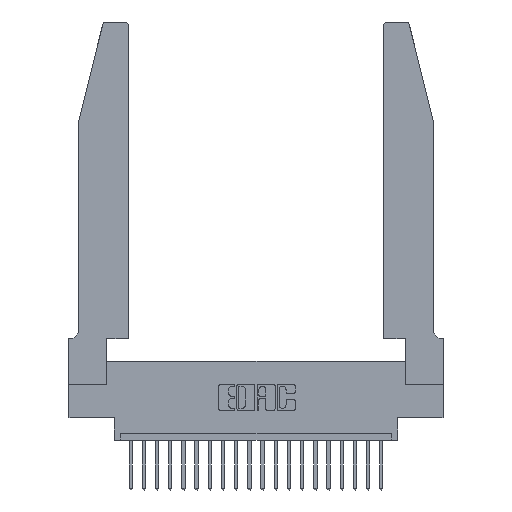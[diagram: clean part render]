
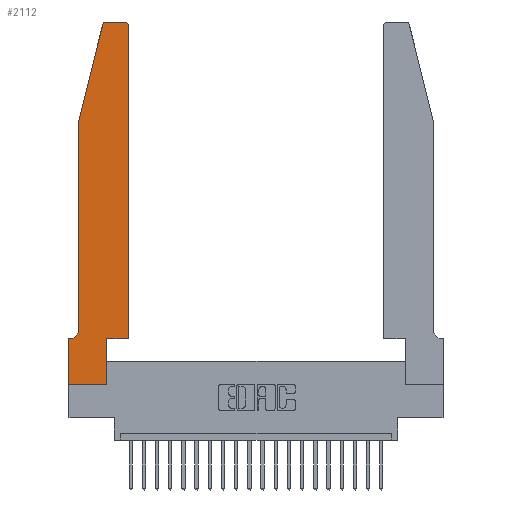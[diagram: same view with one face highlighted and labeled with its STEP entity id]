
A CAD part, top view. The second image highlights one B-rep face of the part: STEP entity #2112.
In plain terms, the highlighted planar face has unit normal (0, 0, 1).
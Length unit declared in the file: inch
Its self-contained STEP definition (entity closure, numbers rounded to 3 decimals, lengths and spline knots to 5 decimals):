
#111 = ORIENTED_EDGE ( 'NONE', *, *, #13829, .T. ) ;
#245 = LINE ( 'NONE', #10132, #5188 ) ;
#274 = CARTESIAN_POINT ( 'NONE',  ( 0.2865, 0., 0.37 ) ) ;
#284 = CIRCLE ( 'NONE', #8115, 0.07 ) ;
#360 = DIRECTION ( 'NONE',  ( -1., 0., 0. ) ) ;
#745 = VERTEX_POINT ( 'NONE', #14329 ) ;
#791 = DIRECTION ( 'NONE',  ( 1., 0., 0. ) ) ;
#1109 = DIRECTION ( 'NONE',  ( 1., 0., 0. ) ) ;
#1461 = CARTESIAN_POINT ( 'NONE',  ( 0.2865, 0.35, 0.37 ) ) ;
#1702 = DIRECTION ( 'NONE',  ( -0.239, -0.971, 0. ) ) ;
#2112 = ADVANCED_FACE ( 'NONE', ( #11909 ), #7901, .T. ) ;
#2151 = DIRECTION ( 'NONE',  ( 0., 1., 0. ) ) ;
#2162 = CARTESIAN_POINT ( 'NONE',  ( 0.25487, 2.72718, 0.37 ) ) ;
#2504 = AXIS2_PLACEMENT_3D ( 'NONE', #12789, #11239, #3029 ) ;
#2702 = VECTOR ( 'NONE', #360, 39.37008 ) ;
#2971 = ORIENTED_EDGE ( 'NONE', *, *, #16387, .T. ) ;
#2990 = CARTESIAN_POINT ( 'NONE',  ( 0.2605, 2.75, 0.37 ) ) ;
#3029 = DIRECTION ( 'NONE',  ( 1., 0., 0. ) ) ;
#3257 = ORIENTED_EDGE ( 'NONE', *, *, #15782, .T. ) ;
#3755 = CARTESIAN_POINT ( 'NONE',  ( 0.4505, 0.35, 0.37 ) ) ;
#3920 = VECTOR ( 'NONE', #17770, 39.37008 ) ;
#4066 = LINE ( 'NONE', #5566, #2702 ) ;
#4079 = LINE ( 'NONE', #17007, #10718 ) ;
#4613 = ORIENTED_EDGE ( 'NONE', *, *, #21035, .T. ) ;
#4940 = CARTESIAN_POINT ( 'NONE',  ( 0., 0.35, 0.37 ) ) ;
#5188 = VECTOR ( 'NONE', #13642, 39.37008 ) ;
#5390 = DIRECTION ( 'NONE',  ( 1., 0., 0. ) ) ;
#5566 = CARTESIAN_POINT ( 'NONE',  ( 0.0755, 0.35, 0.37 ) ) ;
#5670 = VECTOR ( 'NONE', #1702, 39.37008 ) ;
#6150 = VERTEX_POINT ( 'NONE', #6962 ) ;
#6742 = VERTEX_POINT ( 'NONE', #2162 ) ;
#6962 = CARTESIAN_POINT ( 'NONE',  ( 0.0755, 0.42, 0.37 ) ) ;
#7212 = CIRCLE ( 'NONE', #2504, 0.03 ) ;
#7223 = CARTESIAN_POINT ( 'NONE',  ( 0.284, 2.75, 0.37 ) ) ;
#7901 = PLANE ( 'NONE',  #20339 ) ;
#8115 = AXIS2_PLACEMENT_3D ( 'NONE', #10405, #12195, #17314 ) ;
#8593 = EDGE_CURVE ( 'NONE', #9563, #13282, #16603, .T. ) ;
#8942 = CARTESIAN_POINT ( 'NONE',  ( 0.4505, 2.72, 0.37 ) ) ;
#8998 = LINE ( 'NONE', #18800, #5670 ) ;
#9300 = EDGE_CURVE ( 'NONE', #21151, #9563, #21575, .T. ) ;
#9563 = VERTEX_POINT ( 'NONE', #21697 ) ;
#9623 = CARTESIAN_POINT ( 'NONE',  ( 0., 0.35, 0.37 ) ) ;
#9923 = LINE ( 'NONE', #16608, #19365 ) ;
#9980 = CARTESIAN_POINT ( 'NONE',  ( 0., 0., 0.37 ) ) ;
#10132 = CARTESIAN_POINT ( 'NONE',  ( 0., 0., 0.37 ) ) ;
#10140 = EDGE_CURVE ( 'NONE', #19095, #15159, #4079, .T. ) ;
#10267 = ORIENTED_EDGE ( 'NONE', *, *, #9300, .T. ) ;
#10405 = CARTESIAN_POINT ( 'NONE',  ( 0.0055, 0.42, 0.37 ) ) ;
#10718 = VECTOR ( 'NONE', #1109, 39.37008 ) ;
#10751 = ORIENTED_EDGE ( 'NONE', *, *, #13619, .T. ) ;
#11003 = EDGE_CURVE ( 'NONE', #6742, #16909, #8998, .T. ) ;
#11088 = VECTOR ( 'NONE', #5390, 39.37008 ) ;
#11239 = DIRECTION ( 'NONE',  ( 0., 0., 1. ) ) ;
#11283 = VERTEX_POINT ( 'NONE', #4940 ) ;
#11355 = DIRECTION ( 'NONE',  ( 0., 0., 1. ) ) ;
#11592 = CARTESIAN_POINT ( 'NONE',  ( 0.4205, 2.72, 0.37 ) ) ;
#11799 = ORIENTED_EDGE ( 'NONE', *, *, #8593, .T. ) ;
#11909 = FACE_OUTER_BOUND ( 'NONE', #18783, .T. ) ;
#12195 = DIRECTION ( 'NONE',  ( 0., 0., -1. ) ) ;
#12742 = CARTESIAN_POINT ( 'NONE',  ( 0.2865, 0.35, 0.37 ) ) ;
#12754 = VECTOR ( 'NONE', #2151, 39.37008 ) ;
#12789 = CARTESIAN_POINT ( 'NONE',  ( 0.284, 2.72, 0.37 ) ) ;
#13212 = CARTESIAN_POINT ( 'NONE',  ( 0.0755, 2., 0.37 ) ) ;
#13282 = VERTEX_POINT ( 'NONE', #7223 ) ;
#13303 = VECTOR ( 'NONE', #18943, 39.37008 ) ;
#13619 = EDGE_CURVE ( 'NONE', #13282, #6742, #7212, .T. ) ;
#13642 = DIRECTION ( 'NONE',  ( 0., -1., 0. ) ) ;
#13829 = EDGE_CURVE ( 'NONE', #20553, #21151, #20564, .T. ) ;
#14174 = AXIS2_PLACEMENT_3D ( 'NONE', #11592, #18410, #22145 ) ;
#14193 = ORIENTED_EDGE ( 'NONE', *, *, #11003, .T. ) ;
#14329 = CARTESIAN_POINT ( 'NONE',  ( 0.0055, 0.35, 0.37 ) ) ;
#14768 = DIRECTION ( 'NONE',  ( 0., -1., 0. ) ) ;
#15075 = VERTEX_POINT ( 'NONE', #1461 ) ;
#15159 = VERTEX_POINT ( 'NONE', #274 ) ;
#15354 = CARTESIAN_POINT ( 'NONE',  ( 0.4505, 0.35, 0.37 ) ) ;
#15760 = ORIENTED_EDGE ( 'NONE', *, *, #10140, .T. ) ;
#15782 = EDGE_CURVE ( 'NONE', #15075, #20553, #15789, .T. ) ;
#15789 = LINE ( 'NONE', #15863, #11088 ) ;
#15835 = ORIENTED_EDGE ( 'NONE', *, *, #20128, .T. ) ;
#15863 = CARTESIAN_POINT ( 'NONE',  ( 0.4505, 0.35, 0.37 ) ) ;
#16102 = ORIENTED_EDGE ( 'NONE', *, *, #17189, .T. ) ;
#16387 = EDGE_CURVE ( 'NONE', #16909, #6150, #9923, .T. ) ;
#16513 = EDGE_CURVE ( 'NONE', #6150, #745, #284, .T. ) ;
#16603 = LINE ( 'NONE', #2990, #13303 ) ;
#16608 = CARTESIAN_POINT ( 'NONE',  ( 0.0755, 2., 0.37 ) ) ;
#16909 = VERTEX_POINT ( 'NONE', #13212 ) ;
#17007 = CARTESIAN_POINT ( 'NONE',  ( 0., 0., 0.37 ) ) ;
#17189 = EDGE_CURVE ( 'NONE', #745, #11283, #4066, .T. ) ;
#17314 = DIRECTION ( 'NONE',  ( -1., 0., 0. ) ) ;
#17770 = DIRECTION ( 'NONE',  ( 0., 1., 0. ) ) ;
#18410 = DIRECTION ( 'NONE',  ( 0., 0., 1. ) ) ;
#18783 = EDGE_LOOP ( 'NONE', ( #11799, #10751, #14193, #2971, #19239, #16102, #4613, #15760, #15835, #3257, #111, #10267 ) ) ;
#18800 = CARTESIAN_POINT ( 'NONE',  ( 0.0755, 2., 0.37 ) ) ;
#18943 = DIRECTION ( 'NONE',  ( -1., 0., 0. ) ) ;
#19095 = VERTEX_POINT ( 'NONE', #9980 ) ;
#19239 = ORIENTED_EDGE ( 'NONE', *, *, #16513, .T. ) ;
#19365 = VECTOR ( 'NONE', #14768, 39.37008 ) ;
#20128 = EDGE_CURVE ( 'NONE', #15159, #15075, #20767, .T. ) ;
#20339 = AXIS2_PLACEMENT_3D ( 'NONE', #9623, #11355, #791 ) ;
#20553 = VERTEX_POINT ( 'NONE', #15354 ) ;
#20564 = LINE ( 'NONE', #3755, #3920 ) ;
#20767 = LINE ( 'NONE', #12742, #12754 ) ;
#21035 = EDGE_CURVE ( 'NONE', #11283, #19095, #245, .T. ) ;
#21151 = VERTEX_POINT ( 'NONE', #8942 ) ;
#21575 = CIRCLE ( 'NONE', #14174, 0.03 ) ;
#21697 = CARTESIAN_POINT ( 'NONE',  ( 0.4205, 2.75, 0.37 ) ) ;
#22145 = DIRECTION ( 'NONE',  ( 1., 0., 0. ) ) ;
